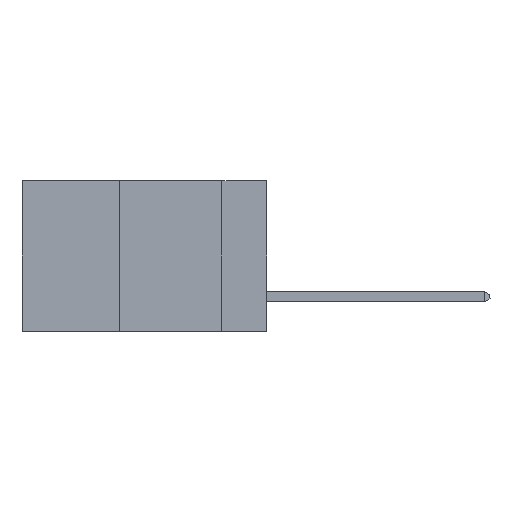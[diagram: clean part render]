
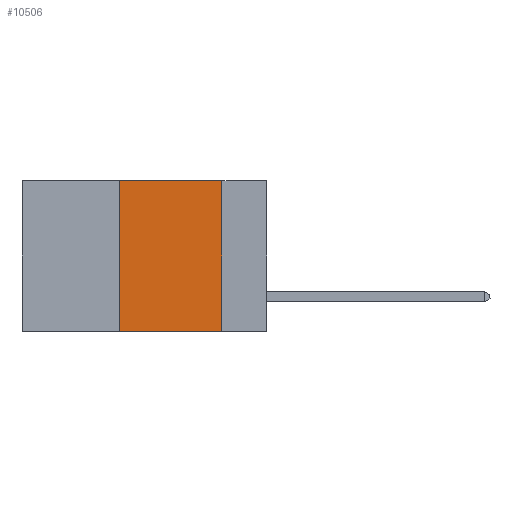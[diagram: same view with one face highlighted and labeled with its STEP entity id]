
A CAD part, left-side view. The second image highlights one B-rep face of the part: STEP entity #10506.
In plain terms, the highlighted planar face has unit normal (-1, 0, 0).
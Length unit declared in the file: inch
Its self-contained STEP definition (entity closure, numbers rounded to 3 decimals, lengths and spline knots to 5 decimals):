
#281 = EDGE_CURVE ( 'NONE', #6048, #8857, #3949, .T. ) ;
#829 = EDGE_CURVE ( 'NONE', #8126, #6654, #5743, .T. ) ;
#949 = VECTOR ( 'NONE', #6110, 39.37008 ) ;
#1421 = CARTESIAN_POINT ( 'NONE',  ( 0., 0.11, 0. ) ) ;
#1584 = CARTESIAN_POINT ( 'NONE',  ( 0., 0.11, -0.37 ) ) ;
#1891 = CARTESIAN_POINT ( 'NONE',  ( 0., 0.6, 0. ) ) ;
#2014 = VECTOR ( 'NONE', #3163, 39.37008 ) ;
#2304 = VECTOR ( 'NONE', #10500, 39.37008 ) ;
#2477 = FACE_OUTER_BOUND ( 'NONE', #3195, .T. ) ;
#3163 = DIRECTION ( 'NONE',  ( 0., 0., -1. ) ) ;
#3195 = EDGE_LOOP ( 'NONE', ( #9406, #6983, #6117, #9537 ) ) ;
#3948 = PLANE ( 'NONE',  #10467 ) ;
#3949 = LINE ( 'NONE', #9346, #2014 ) ;
#5604 = DIRECTION ( 'NONE',  ( 0., 0., -1. ) ) ;
#5635 = CARTESIAN_POINT ( 'NONE',  ( 0., 0.36, 0. ) ) ;
#5642 = CARTESIAN_POINT ( 'NONE',  ( 0., 0.36, 0. ) ) ;
#5743 = LINE ( 'NONE', #5635, #8736 ) ;
#5993 = LINE ( 'NONE', #1891, #949 ) ;
#6048 = VERTEX_POINT ( 'NONE', #1421 ) ;
#6110 = DIRECTION ( 'NONE',  ( 0., -1., 0. ) ) ;
#6117 = ORIENTED_EDGE ( 'NONE', *, *, #829, .F. ) ;
#6317 = CARTESIAN_POINT ( 'NONE',  ( 0., 0.6, -0.37 ) ) ;
#6617 = EDGE_CURVE ( 'NONE', #8126, #8857, #8530, .T. ) ;
#6654 = VERTEX_POINT ( 'NONE', #5642 ) ;
#6683 = CARTESIAN_POINT ( 'NONE',  ( 0., 0.36, -0.37 ) ) ;
#6983 = ORIENTED_EDGE ( 'NONE', *, *, #10238, .F. ) ;
#7210 = DIRECTION ( 'NONE',  ( 1., 0., 0. ) ) ;
#7315 = DIRECTION ( 'NONE',  ( 0., 0., 1. ) ) ;
#8126 = VERTEX_POINT ( 'NONE', #6683 ) ;
#8530 = LINE ( 'NONE', #6317, #2304 ) ;
#8736 = VECTOR ( 'NONE', #7315, 39.37008 ) ;
#8857 = VERTEX_POINT ( 'NONE', #1584 ) ;
#9346 = CARTESIAN_POINT ( 'NONE',  ( 0., 0.11, 0. ) ) ;
#9406 = ORIENTED_EDGE ( 'NONE', *, *, #281, .F. ) ;
#9537 = ORIENTED_EDGE ( 'NONE', *, *, #6617, .T. ) ;
#9642 = CARTESIAN_POINT ( 'NONE',  ( 0., 0.6, 0. ) ) ;
#10238 = EDGE_CURVE ( 'NONE', #6654, #6048, #5993, .T. ) ;
#10467 = AXIS2_PLACEMENT_3D ( 'NONE', #9642, #7210, #5604 ) ;
#10500 = DIRECTION ( 'NONE',  ( 0., -1., 0. ) ) ;
#10506 = ADVANCED_FACE ( 'NONE', ( #2477 ), #3948, .F. ) ;
